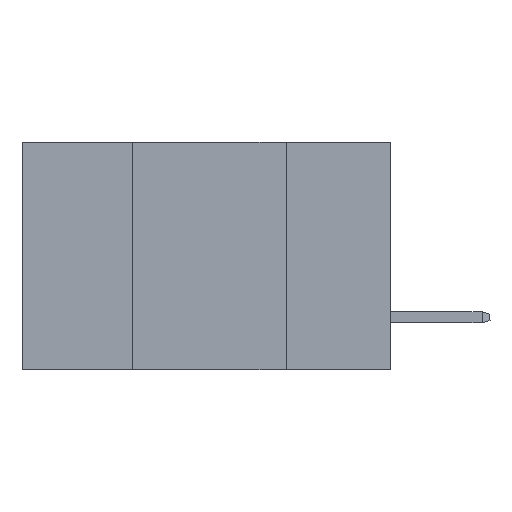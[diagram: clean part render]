
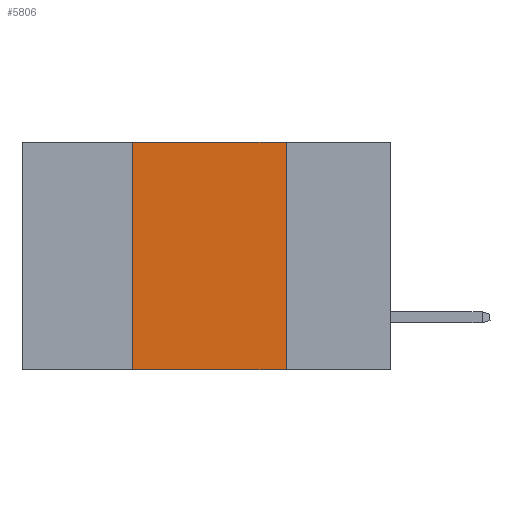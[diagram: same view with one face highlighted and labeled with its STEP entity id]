
A CAD part, left-side view. The second image highlights one B-rep face of the part: STEP entity #5806.
In plain terms, the highlighted planar face has unit normal (-1, 0, 0).
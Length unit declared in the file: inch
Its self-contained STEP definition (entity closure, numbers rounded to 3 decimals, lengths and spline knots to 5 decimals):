
#36 = CARTESIAN_POINT ( 'NONE',  ( 0., 0.6, 0. ) ) ;
#1891 = DIRECTION ( 'NONE',  ( 0., -1., 0. ) ) ;
#2555 = VECTOR ( 'NONE', #5416, 39.37008 ) ;
#3365 = VERTEX_POINT ( 'NONE', #17546 ) ;
#4181 = VERTEX_POINT ( 'NONE', #5116 ) ;
#4548 = LINE ( 'NONE', #9106, #22842 ) ;
#4597 = CARTESIAN_POINT ( 'NONE',  ( 0., 0.17, 0. ) ) ;
#5116 = CARTESIAN_POINT ( 'NONE',  ( 0., 0.42, -0.37 ) ) ;
#5416 = DIRECTION ( 'NONE',  ( 0., 0., -1. ) ) ;
#5806 = ADVANCED_FACE ( 'NONE', ( #7243 ), #23245, .F. ) ;
#6504 = LINE ( 'NONE', #36, #19450 ) ;
#6717 = CARTESIAN_POINT ( 'NONE',  ( 0., 0.42, 0. ) ) ;
#7243 = FACE_OUTER_BOUND ( 'NONE', #16804, .T. ) ;
#7457 = LINE ( 'NONE', #18291, #2555 ) ;
#7943 = ORIENTED_EDGE ( 'NONE', *, *, #17906, .F. ) ;
#8734 = CARTESIAN_POINT ( 'NONE',  ( 0., 0.6, 0. ) ) ;
#9106 = CARTESIAN_POINT ( 'NONE',  ( 0., 0.6, -0.37 ) ) ;
#9234 = VECTOR ( 'NONE', #9509, 39.37008 ) ;
#9509 = DIRECTION ( 'NONE',  ( 0., 0., 1. ) ) ;
#10059 = AXIS2_PLACEMENT_3D ( 'NONE', #8734, #21509, #10614 ) ;
#10544 = EDGE_CURVE ( 'NONE', #12581, #3365, #7457, .T. ) ;
#10614 = DIRECTION ( 'NONE',  ( 0., 0., -1. ) ) ;
#11370 = CARTESIAN_POINT ( 'NONE',  ( 0., 0.42, 0. ) ) ;
#12581 = VERTEX_POINT ( 'NONE', #4597 ) ;
#16585 = ORIENTED_EDGE ( 'NONE', *, *, #10544, .F. ) ;
#16804 = EDGE_LOOP ( 'NONE', ( #16585, #21399, #7943, #17751 ) ) ;
#17546 = CARTESIAN_POINT ( 'NONE',  ( 0., 0.17, -0.37 ) ) ;
#17751 = ORIENTED_EDGE ( 'NONE', *, *, #19567, .T. ) ;
#17906 = EDGE_CURVE ( 'NONE', #4181, #20529, #18991, .T. ) ;
#18291 = CARTESIAN_POINT ( 'NONE',  ( 0., 0.17, 0. ) ) ;
#18991 = LINE ( 'NONE', #11370, #9234 ) ;
#19450 = VECTOR ( 'NONE', #1891, 39.37008 ) ;
#19567 = EDGE_CURVE ( 'NONE', #4181, #3365, #4548, .T. ) ;
#20107 = EDGE_CURVE ( 'NONE', #20529, #12581, #6504, .T. ) ;
#20529 = VERTEX_POINT ( 'NONE', #6717 ) ;
#21399 = ORIENTED_EDGE ( 'NONE', *, *, #20107, .F. ) ;
#21509 = DIRECTION ( 'NONE',  ( 1., 0., 0. ) ) ;
#22842 = VECTOR ( 'NONE', #23674, 39.37008 ) ;
#23245 = PLANE ( 'NONE',  #10059 ) ;
#23674 = DIRECTION ( 'NONE',  ( 0., -1., 0. ) ) ;
